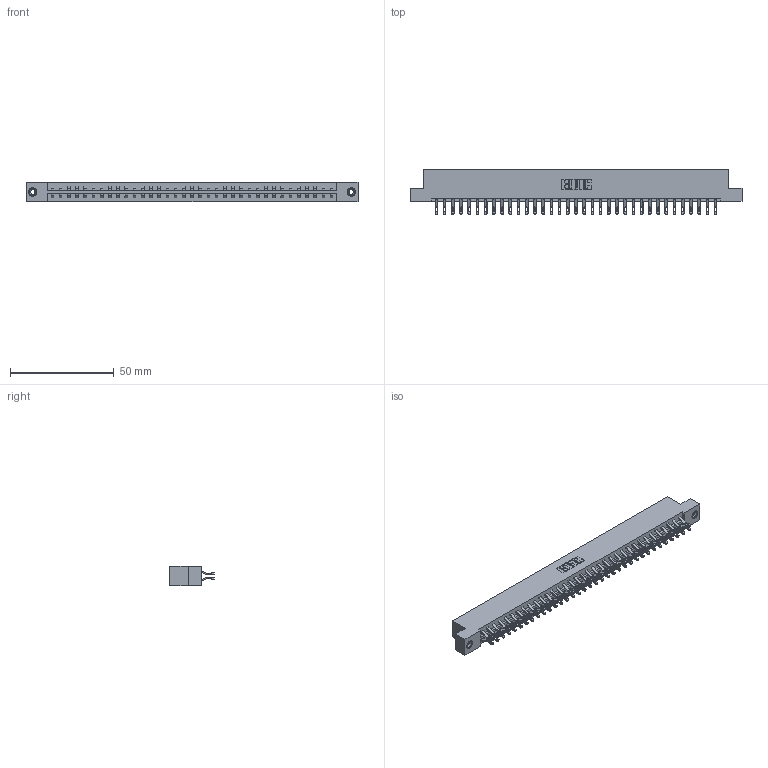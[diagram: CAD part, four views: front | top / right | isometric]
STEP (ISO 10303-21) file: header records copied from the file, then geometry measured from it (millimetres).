
FILE_DESCRIPTION (( 'STEP AP203' ), '1' );
FILE_NAME ('333-070-555-208.STEP', '2018-08-04T15:14:39', ( '' ), ( '' ), 'SwSTEP 2.0', 'SolidWorks 2016', '' );
FILE_SCHEMA (( 'CONFIG_CONTROL_DESIGN' ));
Length unit declared in the file: inch
Products named in the file (4): 333 Part_Flush - .156 Dia - TI; 345-292-001_555 Tail; 345-250-001_345-250-003-102; 333-070-555-208
Assembly tree (73 placements, depth 2):
  333-070-555-208
    333 Part_Flush - .156 Dia - TI
    345-292-001_555 Tail  x70
    345-250-001_345-250-003-102  x2
Bounding box: 160.22 x 21.47 x 9.4 mm (x, y, z)
Volume: 16488.9 mm3; surface area: 20199.9 mm2
Topology: 73 solids, 73 shells, 4234 faces, 13257 edges, 8830 vertices
Faces by surface type: plane 2482, cylinder 1736, cone 12, torus 4
Entity records: 24934 total; most frequent: CARTESIAN_POINT 4159, ORIENTED_EDGE 4058, DIRECTION 3567, EDGE_CURVE 2029, LINE 1861, VECTOR 1861, VERTEX_POINT 1348, AXIS2_PLACEMENT_3D 853
